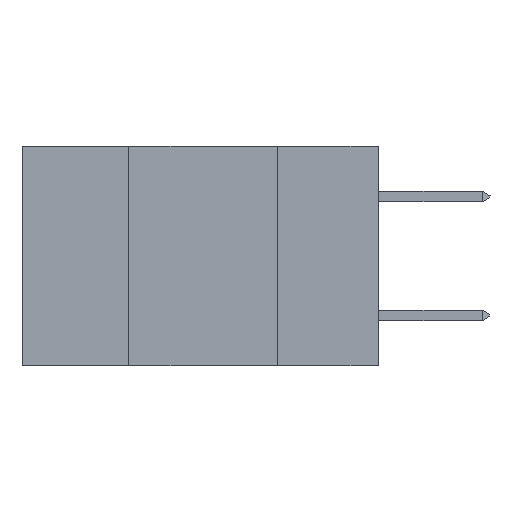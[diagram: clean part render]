
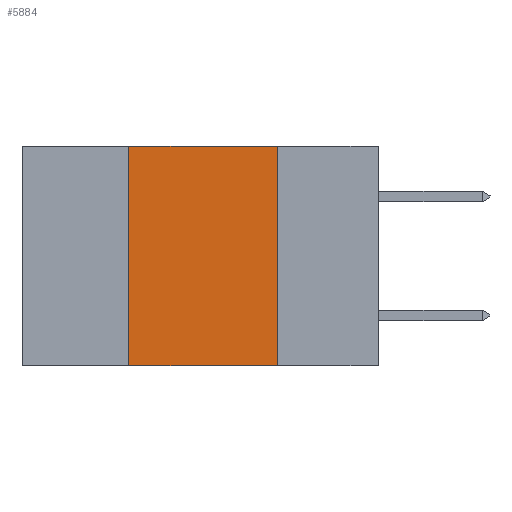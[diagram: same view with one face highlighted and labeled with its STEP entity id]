
A CAD part, left-side view. The second image highlights one B-rep face of the part: STEP entity #5884.
In plain terms, the highlighted planar face has unit normal (-1, 0, 0).
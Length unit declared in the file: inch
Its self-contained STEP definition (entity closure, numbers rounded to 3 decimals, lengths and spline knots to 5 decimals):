
#304 = EDGE_CURVE ( 'NONE', #14743, #16084, #8118, .T. ) ;
#951 = CARTESIAN_POINT ( 'NONE',  ( 0., 0.42, -0.37 ) ) ;
#1611 = EDGE_LOOP ( 'NONE', ( #20165, #1964, #3854, #2457 ) ) ;
#1964 = ORIENTED_EDGE ( 'NONE', *, *, #8048, .F. ) ;
#2457 = ORIENTED_EDGE ( 'NONE', *, *, #304, .T. ) ;
#2554 = DIRECTION ( 'NONE',  ( 1., 0., 0. ) ) ;
#3010 = DIRECTION ( 'NONE',  ( 0., 0., -1. ) ) ;
#3481 = EDGE_CURVE ( 'NONE', #14019, #16084, #13781, .T. ) ;
#3854 = ORIENTED_EDGE ( 'NONE', *, *, #18890, .F. ) ;
#4111 = LINE ( 'NONE', #18502, #13597 ) ;
#5884 = ADVANCED_FACE ( 'NONE', ( #17185 ), #17399, .F. ) ;
#6632 = VECTOR ( 'NONE', #3010, 39.37008 ) ;
#6695 = LINE ( 'NONE', #17426, #19373 ) ;
#8048 = EDGE_CURVE ( 'NONE', #21868, #14019, #6695, .T. ) ;
#8118 = LINE ( 'NONE', #20398, #8535 ) ;
#8535 = VECTOR ( 'NONE', #16970, 39.37008 ) ;
#9766 = CARTESIAN_POINT ( 'NONE',  ( 0., 0.6, 0. ) ) ;
#11888 = DIRECTION ( 'NONE',  ( 0., 0., 1. ) ) ;
#12697 = CARTESIAN_POINT ( 'NONE',  ( 0., 0.17, -0.37 ) ) ;
#13597 = VECTOR ( 'NONE', #11888, 39.37008 ) ;
#13781 = LINE ( 'NONE', #20973, #6632 ) ;
#14019 = VERTEX_POINT ( 'NONE', #14138 ) ;
#14138 = CARTESIAN_POINT ( 'NONE',  ( 0., 0.17, 0. ) ) ;
#14743 = VERTEX_POINT ( 'NONE', #951 ) ;
#16084 = VERTEX_POINT ( 'NONE', #12697 ) ;
#16130 = CARTESIAN_POINT ( 'NONE',  ( 0., 0.42, 0. ) ) ;
#16970 = DIRECTION ( 'NONE',  ( 0., -1., 0. ) ) ;
#17185 = FACE_OUTER_BOUND ( 'NONE', #1611, .T. ) ;
#17399 = PLANE ( 'NONE',  #17483 ) ;
#17426 = CARTESIAN_POINT ( 'NONE',  ( 0., 0.6, 0. ) ) ;
#17483 = AXIS2_PLACEMENT_3D ( 'NONE', #9766, #2554, #22401 ) ;
#18502 = CARTESIAN_POINT ( 'NONE',  ( 0., 0.42, -0.37 ) ) ;
#18890 = EDGE_CURVE ( 'NONE', #14743, #21868, #4111, .T. ) ;
#19373 = VECTOR ( 'NONE', #19436, 39.37008 ) ;
#19436 = DIRECTION ( 'NONE',  ( 0., -1., 0. ) ) ;
#20165 = ORIENTED_EDGE ( 'NONE', *, *, #3481, .F. ) ;
#20398 = CARTESIAN_POINT ( 'NONE',  ( 0., 0.6, -0.37 ) ) ;
#20973 = CARTESIAN_POINT ( 'NONE',  ( 0., 0.17, -0.37 ) ) ;
#21868 = VERTEX_POINT ( 'NONE', #16130 ) ;
#22401 = DIRECTION ( 'NONE',  ( 0., 0., -1. ) ) ;
